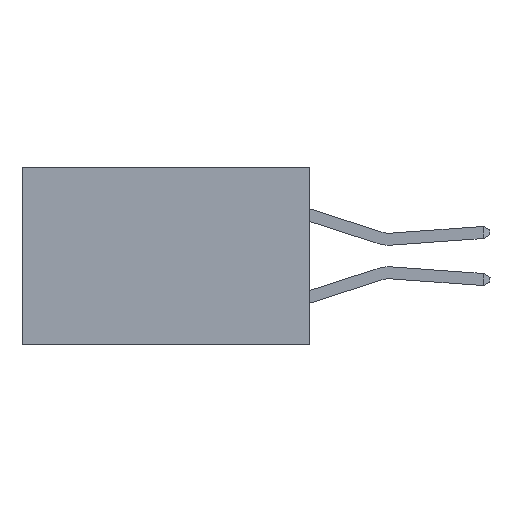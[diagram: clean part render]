
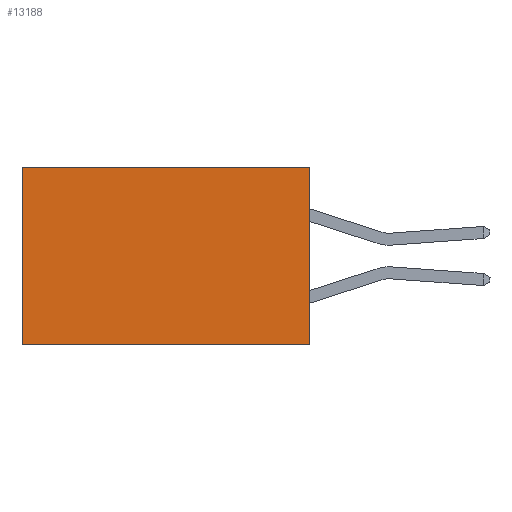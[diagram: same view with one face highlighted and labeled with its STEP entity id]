
A CAD part, left-side view. The second image highlights one B-rep face of the part: STEP entity #13188.
In plain terms, the highlighted planar face has unit normal (-1, 0, 0).
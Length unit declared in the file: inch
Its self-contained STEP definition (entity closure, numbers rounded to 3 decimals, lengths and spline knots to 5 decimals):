
#1793 = CARTESIAN_POINT ( 'NONE',  ( 0.298, 0., 0. ) ) ;
#2230 = DIRECTION ( 'NONE',  ( 0., 0., -1. ) ) ;
#3865 = EDGE_CURVE ( 'NONE', #9524, #25237, #18279, .T. ) ;
#4514 = DIRECTION ( 'NONE',  ( 1., 0., 0. ) ) ;
#5687 = CARTESIAN_POINT ( 'NONE',  ( 0.298, 0., 0. ) ) ;
#6685 = DIRECTION ( 'NONE',  ( 0., 0., -1. ) ) ;
#9524 = VERTEX_POINT ( 'NONE', #25993 ) ;
#10114 = EDGE_CURVE ( 'NONE', #12564, #25237, #10769, .T. ) ;
#10239 = VERTEX_POINT ( 'NONE', #23208 ) ;
#10351 = FACE_OUTER_BOUND ( 'NONE', #25424, .T. ) ;
#10769 = LINE ( 'NONE', #16731, #11865 ) ;
#10901 = VECTOR ( 'NONE', #2230, 39.37008 ) ;
#11749 = DIRECTION ( 'NONE',  ( 0., 0., -1. ) ) ;
#11865 = VECTOR ( 'NONE', #21239, 39.37008 ) ;
#12564 = VERTEX_POINT ( 'NONE', #15327 ) ;
#13188 = ADVANCED_FACE ( 'NONE', ( #10351 ), #30198, .F. ) ;
#15327 = CARTESIAN_POINT ( 'NONE',  ( 0.298, 0., -0.37 ) ) ;
#15398 = DIRECTION ( 'NONE',  ( 0., 1., 0. ) ) ;
#15601 = LINE ( 'NONE', #1793, #23344 ) ;
#16731 = CARTESIAN_POINT ( 'NONE',  ( 0.298, 0., -0.37 ) ) ;
#17412 = VECTOR ( 'NONE', #15398, 39.37008 ) ;
#18279 = LINE ( 'NONE', #25884, #10901 ) ;
#18672 = CARTESIAN_POINT ( 'NONE',  ( 0.298, 0.6, -0.37 ) ) ;
#18949 = ORIENTED_EDGE ( 'NONE', *, *, #28912, .F. ) ;
#20776 = ORIENTED_EDGE ( 'NONE', *, *, #10114, .F. ) ;
#21239 = DIRECTION ( 'NONE',  ( 0., 1., 0. ) ) ;
#23208 = CARTESIAN_POINT ( 'NONE',  ( 0.298, 0., 0. ) ) ;
#23344 = VECTOR ( 'NONE', #6685, 39.37008 ) ;
#23501 = CARTESIAN_POINT ( 'NONE',  ( 0.298, 0., 0. ) ) ;
#25237 = VERTEX_POINT ( 'NONE', #18672 ) ;
#25424 = EDGE_LOOP ( 'NONE', ( #29879, #20776, #18949, #28904 ) ) ;
#25512 = AXIS2_PLACEMENT_3D ( 'NONE', #23501, #4514, #11749 ) ;
#25884 = CARTESIAN_POINT ( 'NONE',  ( 0.298, 0.6, 0. ) ) ;
#25993 = CARTESIAN_POINT ( 'NONE',  ( 0.298, 0.6, 0. ) ) ;
#28406 = LINE ( 'NONE', #5687, #17412 ) ;
#28904 = ORIENTED_EDGE ( 'NONE', *, *, #30272, .T. ) ;
#28912 = EDGE_CURVE ( 'NONE', #10239, #12564, #15601, .T. ) ;
#29879 = ORIENTED_EDGE ( 'NONE', *, *, #3865, .T. ) ;
#30198 = PLANE ( 'NONE',  #25512 ) ;
#30272 = EDGE_CURVE ( 'NONE', #10239, #9524, #28406, .T. ) ;
